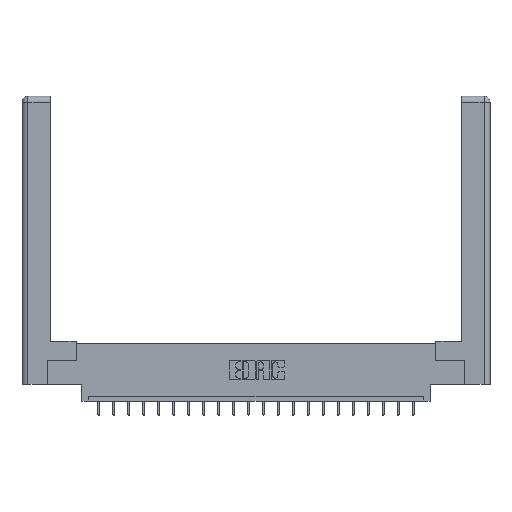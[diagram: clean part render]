
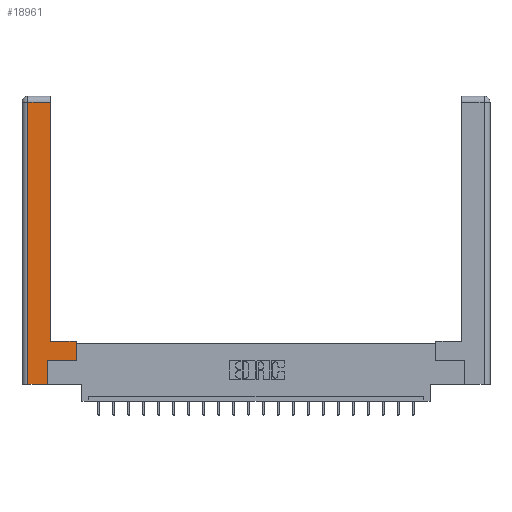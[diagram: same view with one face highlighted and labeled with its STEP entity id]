
A CAD part, top view. The second image highlights one B-rep face of the part: STEP entity #18961.
In plain terms, the highlighted planar face has unit normal (0, 0, 1).
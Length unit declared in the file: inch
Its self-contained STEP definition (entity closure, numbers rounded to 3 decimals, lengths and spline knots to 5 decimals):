
#598 = ORIENTED_EDGE ( 'NONE', *, *, #4135, .T. ) ;
#735 = ORIENTED_EDGE ( 'NONE', *, *, #14718, .T. ) ;
#1761 = VERTEX_POINT ( 'NONE', #21508 ) ;
#2333 = LINE ( 'NONE', #21136, #19614 ) ;
#2359 = CARTESIAN_POINT ( 'NONE',  ( 0.0615, 0., 0. ) ) ;
#2555 = DIRECTION ( 'NONE',  ( 0., -1., 0. ) ) ;
#3229 = CARTESIAN_POINT ( 'NONE',  ( 0.295, 0.45, 0. ) ) ;
#3610 = DIRECTION ( 'NONE',  ( 0., 1., 0. ) ) ;
#3711 = CARTESIAN_POINT ( 'NONE',  ( 0.265, 0.245, 0. ) ) ;
#4135 = EDGE_CURVE ( 'NONE', #14253, #8200, #12661, .T. ) ;
#4443 = VERTEX_POINT ( 'NONE', #10699 ) ;
#4960 = DIRECTION ( 'NONE',  ( 1., 0., 0. ) ) ;
#5209 = VECTOR ( 'NONE', #19615, 39.37008 ) ;
#5496 = LINE ( 'NONE', #3229, #13909 ) ;
#5919 = CARTESIAN_POINT ( 'NONE',  ( 0.265, 0., 0. ) ) ;
#6535 = DIRECTION ( 'NONE',  ( -1., 0., 0. ) ) ;
#6732 = VERTEX_POINT ( 'NONE', #3711 ) ;
#6999 = CARTESIAN_POINT ( 'NONE',  ( 0.565, 0.245, 0. ) ) ;
#7381 = ORIENTED_EDGE ( 'NONE', *, *, #8799, .T. ) ;
#7395 = VERTEX_POINT ( 'NONE', #19993 ) ;
#8200 = VERTEX_POINT ( 'NONE', #18923 ) ;
#8343 = EDGE_CURVE ( 'NONE', #8200, #4443, #5496, .T. ) ;
#8642 = LINE ( 'NONE', #5919, #17293 ) ;
#8799 = EDGE_CURVE ( 'NONE', #20009, #21423, #20727, .T. ) ;
#9147 = EDGE_CURVE ( 'NONE', #4443, #20009, #2333, .T. ) ;
#9883 = DIRECTION ( 'NONE',  ( 0., 1., 0. ) ) ;
#9887 = ORIENTED_EDGE ( 'NONE', *, *, #10467, .T. ) ;
#10257 = CARTESIAN_POINT ( 'NONE',  ( 0., 0., 0. ) ) ;
#10358 = FACE_OUTER_BOUND ( 'NONE', #21522, .T. ) ;
#10467 = EDGE_CURVE ( 'NONE', #6732, #14253, #11170, .T. ) ;
#10699 = CARTESIAN_POINT ( 'NONE',  ( 0.295, 0.45, 0. ) ) ;
#10732 = LINE ( 'NONE', #19985, #14337 ) ;
#10864 = VECTOR ( 'NONE', #3610, 39.37008 ) ;
#11007 = DIRECTION ( 'NONE',  ( 1., 0., 0. ) ) ;
#11170 = LINE ( 'NONE', #16542, #11951 ) ;
#11699 = DIRECTION ( 'NONE',  ( 0., 0., -1. ) ) ;
#11724 = CARTESIAN_POINT ( 'NONE',  ( 0.0615, 2.94, 0. ) ) ;
#11951 = VECTOR ( 'NONE', #4960, 39.37008 ) ;
#12571 = LINE ( 'NONE', #2359, #19133 ) ;
#12661 = LINE ( 'NONE', #13805, #10864 ) ;
#13805 = CARTESIAN_POINT ( 'NONE',  ( 0.565, 0.45, 0. ) ) ;
#13909 = VECTOR ( 'NONE', #6535, 39.37008 ) ;
#14040 = CARTESIAN_POINT ( 'NONE',  ( 0.295, 2.94, 0. ) ) ;
#14253 = VERTEX_POINT ( 'NONE', #6999 ) ;
#14337 = VECTOR ( 'NONE', #9883, 39.37008 ) ;
#14637 = CARTESIAN_POINT ( 'NONE',  ( 0.0615, 2.94, 0. ) ) ;
#14718 = EDGE_CURVE ( 'NONE', #21423, #1761, #12571, .T. ) ;
#14805 = EDGE_CURVE ( 'NONE', #1761, #7395, #8642, .T. ) ;
#15060 = DIRECTION ( 'NONE',  ( -1., 0., 0. ) ) ;
#15952 = ORIENTED_EDGE ( 'NONE', *, *, #14805, .T. ) ;
#16542 = CARTESIAN_POINT ( 'NONE',  ( 0.565, 0.245, 0. ) ) ;
#17272 = EDGE_CURVE ( 'NONE', #7395, #6732, #10732, .T. ) ;
#17293 = VECTOR ( 'NONE', #11007, 39.37008 ) ;
#18923 = CARTESIAN_POINT ( 'NONE',  ( 0.565, 0.45, 0. ) ) ;
#18961 = ADVANCED_FACE ( 'NONE', ( #10358 ), #21714, .F. ) ;
#19133 = VECTOR ( 'NONE', #2555, 39.37008 ) ;
#19237 = DIRECTION ( 'NONE',  ( 0., 1., 0. ) ) ;
#19614 = VECTOR ( 'NONE', #19237, 39.37008 ) ;
#19615 = DIRECTION ( 'NONE',  ( -1., 0., 0. ) ) ;
#19985 = CARTESIAN_POINT ( 'NONE',  ( 0.265, 0.245, 0. ) ) ;
#19993 = CARTESIAN_POINT ( 'NONE',  ( 0.265, 0., 0. ) ) ;
#20009 = VERTEX_POINT ( 'NONE', #14040 ) ;
#20178 = ORIENTED_EDGE ( 'NONE', *, *, #8343, .T. ) ;
#20727 = LINE ( 'NONE', #14637, #5209 ) ;
#20815 = AXIS2_PLACEMENT_3D ( 'NONE', #10257, #11699, #15060 ) ;
#20980 = ORIENTED_EDGE ( 'NONE', *, *, #17272, .T. ) ;
#21136 = CARTESIAN_POINT ( 'NONE',  ( 0.295, 3., 0. ) ) ;
#21333 = ORIENTED_EDGE ( 'NONE', *, *, #9147, .T. ) ;
#21423 = VERTEX_POINT ( 'NONE', #11724 ) ;
#21508 = CARTESIAN_POINT ( 'NONE',  ( 0.0615, 0., 0. ) ) ;
#21522 = EDGE_LOOP ( 'NONE', ( #21333, #7381, #735, #15952, #20980, #9887, #598, #20178 ) ) ;
#21714 = PLANE ( 'NONE',  #20815 ) ;
